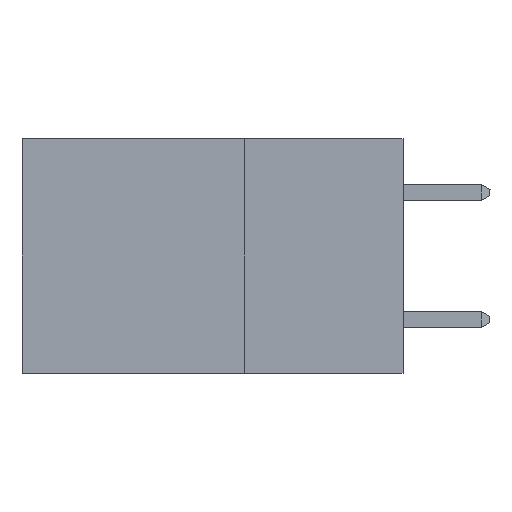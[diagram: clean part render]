
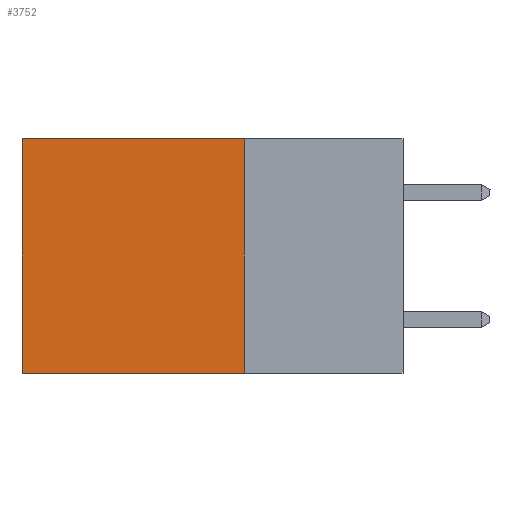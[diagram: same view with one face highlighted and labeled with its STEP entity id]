
A CAD part, left-side view. The second image highlights one B-rep face of the part: STEP entity #3752.
In plain terms, the highlighted planar face has unit normal (-1, 0, 0).
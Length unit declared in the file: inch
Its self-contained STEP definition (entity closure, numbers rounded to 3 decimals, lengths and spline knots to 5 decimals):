
#672 = ORIENTED_EDGE ( 'NONE', *, *, #12627, .F. ) ;
#1008 = CARTESIAN_POINT ( 'NONE',  ( 0.2875, 0.25, -0.37 ) ) ;
#1311 = ORIENTED_EDGE ( 'NONE', *, *, #7128, .F. ) ;
#1604 = ORIENTED_EDGE ( 'NONE', *, *, #10771, .T. ) ;
#1655 = EDGE_CURVE ( 'NONE', #2687, #2916, #6090, .T. ) ;
#2232 = LINE ( 'NONE', #1008, #2854 ) ;
#2363 = CARTESIAN_POINT ( 'NONE',  ( 0.2875, 0.6, 0. ) ) ;
#2680 = LINE ( 'NONE', #7010, #3283 ) ;
#2687 = VERTEX_POINT ( 'NONE', #12452 ) ;
#2854 = VECTOR ( 'NONE', #4916, 39.37008 ) ;
#2916 = VERTEX_POINT ( 'NONE', #2363 ) ;
#2960 = CARTESIAN_POINT ( 'NONE',  ( 0.2875, 0.25, -0.37 ) ) ;
#3197 = CARTESIAN_POINT ( 'NONE',  ( 0.2875, 0.25, 0. ) ) ;
#3283 = VECTOR ( 'NONE', #9041, 39.37008 ) ;
#3752 = ADVANCED_FACE ( 'NONE', ( #12634 ), #4184, .F. ) ;
#4184 = PLANE ( 'NONE',  #7256 ) ;
#4702 = DIRECTION ( 'NONE',  ( 0., 1., 0. ) ) ;
#4916 = DIRECTION ( 'NONE',  ( 0., 1., 0. ) ) ;
#6090 = LINE ( 'NONE', #3197, #7045 ) ;
#6687 = EDGE_LOOP ( 'NONE', ( #1604, #1311, #672, #8074 ) ) ;
#7010 = CARTESIAN_POINT ( 'NONE',  ( 0.2875, 0.25, 0. ) ) ;
#7045 = VECTOR ( 'NONE', #4702, 39.37008 ) ;
#7128 = EDGE_CURVE ( 'NONE', #10453, #9380, #2232, .T. ) ;
#7256 = AXIS2_PLACEMENT_3D ( 'NONE', #11114, #9261, #8073 ) ;
#8073 = DIRECTION ( 'NONE',  ( 0., 0., -1. ) ) ;
#8074 = ORIENTED_EDGE ( 'NONE', *, *, #1655, .T. ) ;
#8160 = DIRECTION ( 'NONE',  ( 0., 0., -1. ) ) ;
#8460 = LINE ( 'NONE', #11166, #11289 ) ;
#9041 = DIRECTION ( 'NONE',  ( 0., 0., -1. ) ) ;
#9261 = DIRECTION ( 'NONE',  ( 1., 0., 0. ) ) ;
#9380 = VERTEX_POINT ( 'NONE', #10532 ) ;
#10453 = VERTEX_POINT ( 'NONE', #2960 ) ;
#10532 = CARTESIAN_POINT ( 'NONE',  ( 0.2875, 0.6, -0.37 ) ) ;
#10771 = EDGE_CURVE ( 'NONE', #2916, #9380, #8460, .T. ) ;
#11114 = CARTESIAN_POINT ( 'NONE',  ( 0.2875, 0.25, 0. ) ) ;
#11166 = CARTESIAN_POINT ( 'NONE',  ( 0.2875, 0.6, 0. ) ) ;
#11289 = VECTOR ( 'NONE', #8160, 39.37008 ) ;
#12452 = CARTESIAN_POINT ( 'NONE',  ( 0.2875, 0.25, 0. ) ) ;
#12627 = EDGE_CURVE ( 'NONE', #2687, #10453, #2680, .T. ) ;
#12634 = FACE_OUTER_BOUND ( 'NONE', #6687, .T. ) ;
